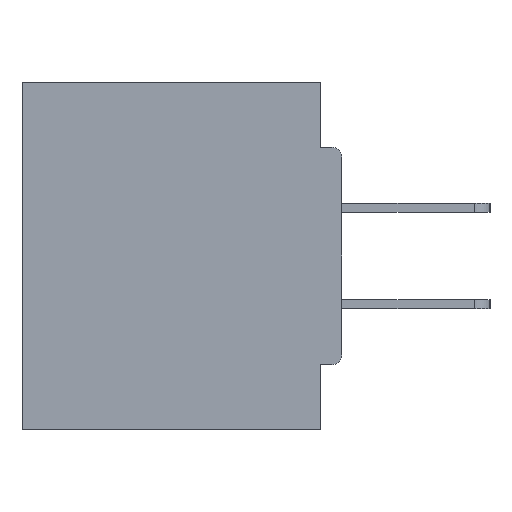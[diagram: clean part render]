
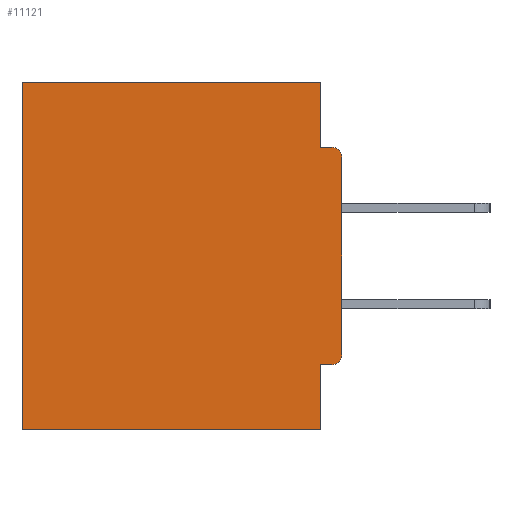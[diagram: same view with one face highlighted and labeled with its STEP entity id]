
A CAD part, left-side view. The second image highlights one B-rep face of the part: STEP entity #11121.
In plain terms, the highlighted planar face has unit normal (-1, 0, 0).
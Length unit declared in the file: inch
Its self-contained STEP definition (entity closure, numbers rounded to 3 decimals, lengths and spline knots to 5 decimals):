
#528 = CARTESIAN_POINT ( 'NONE',  ( 0.298, 0.015, -0.1085 ) ) ;
#1091 = VECTOR ( 'NONE', #23168, 39.37008 ) ;
#1264 = VECTOR ( 'NONE', #32423, 39.37008 ) ;
#2839 = VERTEX_POINT ( 'NONE', #4877 ) ;
#3006 = CARTESIAN_POINT ( 'NONE',  ( 0.298, 0.031, 0. ) ) ;
#4824 = VECTOR ( 'NONE', #29503, 39.37008 ) ;
#4877 = CARTESIAN_POINT ( 'NONE',  ( 0.298, 0., -0.3915 ) ) ;
#5252 = VERTEX_POINT ( 'NONE', #15579 ) ;
#5567 = DIRECTION ( 'NONE',  ( -1., 0., 0. ) ) ;
#5796 = VERTEX_POINT ( 'NONE', #24933 ) ;
#6642 = VERTEX_POINT ( 'NONE', #27352 ) ;
#6684 = DIRECTION ( 'NONE',  ( 0., 0., -1. ) ) ;
#6814 = EDGE_CURVE ( 'NONE', #23613, #13732, #36734, .T. ) ;
#7491 = DIRECTION ( 'NONE',  ( 0., 0., -1. ) ) ;
#7620 = EDGE_CURVE ( 'NONE', #21393, #5796, #26025, .T. ) ;
#7622 = CARTESIAN_POINT ( 'NONE',  ( 0.298, 0.46, 0. ) ) ;
#8328 = ORIENTED_EDGE ( 'NONE', *, *, #28982, .F. ) ;
#9834 = CARTESIAN_POINT ( 'NONE',  ( 0.298, 0.031, -0.5 ) ) ;
#10019 = CARTESIAN_POINT ( 'NONE',  ( 0.298, 0.46, -0.5 ) ) ;
#10067 = LINE ( 'NONE', #9834, #30890 ) ;
#10104 = EDGE_CURVE ( 'NONE', #35406, #6642, #14608, .T. ) ;
#11121 = ADVANCED_FACE ( 'NONE', ( #37262 ), #24725, .F. ) ;
#11403 = DIRECTION ( 'NONE',  ( 0., 0., -1. ) ) ;
#13647 = LINE ( 'NONE', #20155, #4824 ) ;
#13732 = VERTEX_POINT ( 'NONE', #10019 ) ;
#14180 = ORIENTED_EDGE ( 'NONE', *, *, #24333, .T. ) ;
#14252 = EDGE_CURVE ( 'NONE', #5252, #33904, #15792, .T. ) ;
#14608 = LINE ( 'NONE', #26913, #18716 ) ;
#15504 = EDGE_CURVE ( 'NONE', #21393, #2839, #28170, .T. ) ;
#15579 = CARTESIAN_POINT ( 'NONE',  ( 0.298, 0., -0.1085 ) ) ;
#15792 = CIRCLE ( 'NONE', #31039, 0.015 ) ;
#16305 = VECTOR ( 'NONE', #7491, 39.37008 ) ;
#16354 = VECTOR ( 'NONE', #22925, 39.37008 ) ;
#18158 = CARTESIAN_POINT ( 'NONE',  ( 0.298, 0.031, -0.0935 ) ) ;
#18243 = DIRECTION ( 'NONE',  ( 0., 1., 0. ) ) ;
#18383 = EDGE_CURVE ( 'NONE', #33028, #33904, #27956, .T. ) ;
#18716 = VECTOR ( 'NONE', #18243, 39.37008 ) ;
#18801 = ORIENTED_EDGE ( 'NONE', *, *, #21279, .F. ) ;
#18823 = LINE ( 'NONE', #32539, #1264 ) ;
#20155 = CARTESIAN_POINT ( 'NONE',  ( 0.298, 0., 0. ) ) ;
#20287 = CARTESIAN_POINT ( 'NONE',  ( 0.298, 0.015, -0.3915 ) ) ;
#20453 = ORIENTED_EDGE ( 'NONE', *, *, #10104, .T. ) ;
#21169 = DIRECTION ( 'NONE',  ( -1., 0., 0. ) ) ;
#21279 = EDGE_CURVE ( 'NONE', #35406, #33028, #10067, .T. ) ;
#21393 = VERTEX_POINT ( 'NONE', #37387 ) ;
#21623 = DIRECTION ( 'NONE',  ( 1., 0., 0. ) ) ;
#21870 = VECTOR ( 'NONE', #28403, 39.37008 ) ;
#22178 = ORIENTED_EDGE ( 'NONE', *, *, #18383, .F. ) ;
#22305 = ORIENTED_EDGE ( 'NONE', *, *, #15504, .T. ) ;
#22925 = DIRECTION ( 'NONE',  ( 0., -1., 0. ) ) ;
#23168 = DIRECTION ( 'NONE',  ( 0., 1., 0. ) ) ;
#23613 = VERTEX_POINT ( 'NONE', #24136 ) ;
#24136 = CARTESIAN_POINT ( 'NONE',  ( 0.298, 0.031, -0.5 ) ) ;
#24333 = EDGE_CURVE ( 'NONE', #6642, #13732, #37661, .T. ) ;
#24725 = PLANE ( 'NONE',  #33802 ) ;
#24892 = DIRECTION ( 'NONE',  ( 0., 0., -1. ) ) ;
#24933 = CARTESIAN_POINT ( 'NONE',  ( 0.298, 0.031, -0.4065 ) ) ;
#25372 = CARTESIAN_POINT ( 'NONE',  ( 0.298, 0., -0.5 ) ) ;
#25520 = CARTESIAN_POINT ( 'NONE',  ( 0.298, 0., -0.0935 ) ) ;
#26025 = LINE ( 'NONE', #32152, #1091 ) ;
#26913 = CARTESIAN_POINT ( 'NONE',  ( 0.298, 0., 0. ) ) ;
#27352 = CARTESIAN_POINT ( 'NONE',  ( 0.298, 0.46, 0. ) ) ;
#27468 = CARTESIAN_POINT ( 'NONE',  ( 0.298, 0., 0. ) ) ;
#27956 = LINE ( 'NONE', #25520, #16354 ) ;
#28170 = CIRCLE ( 'NONE', #34766, 0.015 ) ;
#28403 = DIRECTION ( 'NONE',  ( 0., 1., 0. ) ) ;
#28982 = EDGE_CURVE ( 'NONE', #5252, #2839, #13647, .T. ) ;
#29503 = DIRECTION ( 'NONE',  ( 0., 0., -1. ) ) ;
#30890 = VECTOR ( 'NONE', #24892, 39.37008 ) ;
#31039 = AXIS2_PLACEMENT_3D ( 'NONE', #528, #21169, #36480 ) ;
#31308 = ORIENTED_EDGE ( 'NONE', *, *, #14252, .T. ) ;
#32152 = CARTESIAN_POINT ( 'NONE',  ( 0.298, 0., -0.4065 ) ) ;
#32423 = DIRECTION ( 'NONE',  ( 0., 0., -1. ) ) ;
#32539 = CARTESIAN_POINT ( 'NONE',  ( 0.298, 0.031, -0.5 ) ) ;
#32630 = ORIENTED_EDGE ( 'NONE', *, *, #6814, .F. ) ;
#33028 = VERTEX_POINT ( 'NONE', #18158 ) ;
#33802 = AXIS2_PLACEMENT_3D ( 'NONE', #27468, #21623, #6684 ) ;
#33904 = VERTEX_POINT ( 'NONE', #37546 ) ;
#34766 = AXIS2_PLACEMENT_3D ( 'NONE', #20287, #5567, #11403 ) ;
#35172 = EDGE_LOOP ( 'NONE', ( #31308, #22178, #18801, #20453, #14180, #32630, #37144, #37671, #22305, #8328 ) ) ;
#35406 = VERTEX_POINT ( 'NONE', #3006 ) ;
#36480 = DIRECTION ( 'NONE',  ( 0., 0., -1. ) ) ;
#36734 = LINE ( 'NONE', #25372, #21870 ) ;
#37144 = ORIENTED_EDGE ( 'NONE', *, *, #38064, .F. ) ;
#37262 = FACE_OUTER_BOUND ( 'NONE', #35172, .T. ) ;
#37387 = CARTESIAN_POINT ( 'NONE',  ( 0.298, 0.015, -0.4065 ) ) ;
#37546 = CARTESIAN_POINT ( 'NONE',  ( 0.298, 0.015, -0.0935 ) ) ;
#37661 = LINE ( 'NONE', #7622, #16305 ) ;
#37671 = ORIENTED_EDGE ( 'NONE', *, *, #7620, .F. ) ;
#38064 = EDGE_CURVE ( 'NONE', #5796, #23613, #18823, .T. ) ;
